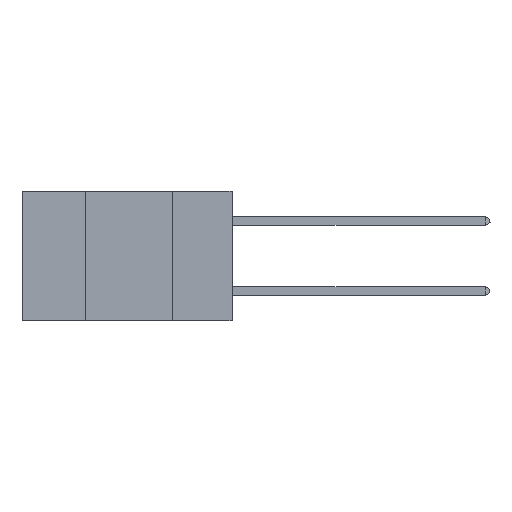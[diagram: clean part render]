
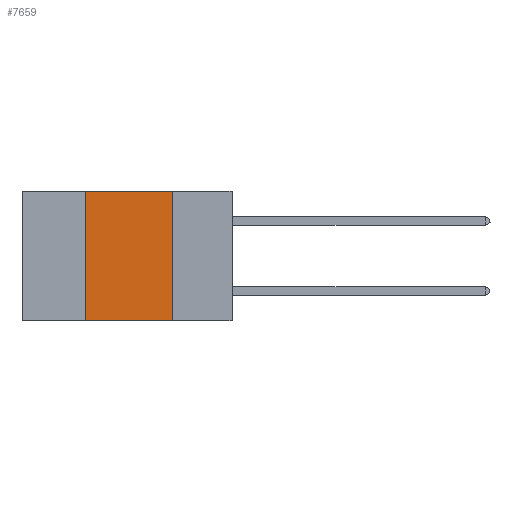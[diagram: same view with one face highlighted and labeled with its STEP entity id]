
A CAD part, left-side view. The second image highlights one B-rep face of the part: STEP entity #7659.
In plain terms, the highlighted planar face has unit normal (-1, 0, 0).
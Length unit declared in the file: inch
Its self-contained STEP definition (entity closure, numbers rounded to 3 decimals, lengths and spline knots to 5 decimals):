
#226 = DIRECTION ( 'NONE',  ( 0., 0., -1. ) ) ;
#374 = ORIENTED_EDGE ( 'NONE', *, *, #7671, .F. ) ;
#540 = VERTEX_POINT ( 'NONE', #12901 ) ;
#922 = EDGE_LOOP ( 'NONE', ( #374, #12411, #3783, #12778 ) ) ;
#1341 = LINE ( 'NONE', #3251, #9674 ) ;
#1402 = CARTESIAN_POINT ( 'NONE',  ( 0., 0.17, 0. ) ) ;
#3251 = CARTESIAN_POINT ( 'NONE',  ( 0., 0.42, 0. ) ) ;
#3254 = VECTOR ( 'NONE', #10732, 39.37008 ) ;
#3783 = ORIENTED_EDGE ( 'NONE', *, *, #9720, .F. ) ;
#4323 = DIRECTION ( 'NONE',  ( 0., 0., 1. ) ) ;
#4763 = DIRECTION ( 'NONE',  ( 1., 0., 0. ) ) ;
#4970 = VERTEX_POINT ( 'NONE', #5935 ) ;
#5128 = LINE ( 'NONE', #1402, #10412 ) ;
#5935 = CARTESIAN_POINT ( 'NONE',  ( 0., 0.17, 0. ) ) ;
#6244 = LINE ( 'NONE', #14028, #3254 ) ;
#6791 = CARTESIAN_POINT ( 'NONE',  ( 0., 0.6, 0. ) ) ;
#7073 = CARTESIAN_POINT ( 'NONE',  ( 0., 0.42, 0. ) ) ;
#7356 = CARTESIAN_POINT ( 'NONE',  ( 0., 0.42, -0.37 ) ) ;
#7659 = ADVANCED_FACE ( 'NONE', ( #13411 ), #11521, .F. ) ;
#7670 = VECTOR ( 'NONE', #11267, 39.37008 ) ;
#7671 = EDGE_CURVE ( 'NONE', #4970, #540, #5128, .T. ) ;
#7814 = VERTEX_POINT ( 'NONE', #7356 ) ;
#8778 = VERTEX_POINT ( 'NONE', #7073 ) ;
#9674 = VECTOR ( 'NONE', #4323, 39.37008 ) ;
#9720 = EDGE_CURVE ( 'NONE', #7814, #8778, #1341, .T. ) ;
#10387 = CARTESIAN_POINT ( 'NONE',  ( 0., 0.6, 0. ) ) ;
#10412 = VECTOR ( 'NONE', #226, 39.37008 ) ;
#10634 = LINE ( 'NONE', #6791, #7670 ) ;
#10732 = DIRECTION ( 'NONE',  ( 0., -1., 0. ) ) ;
#10953 = AXIS2_PLACEMENT_3D ( 'NONE', #10387, #4763, #12661 ) ;
#11267 = DIRECTION ( 'NONE',  ( 0., -1., 0. ) ) ;
#11521 = PLANE ( 'NONE',  #10953 ) ;
#12231 = EDGE_CURVE ( 'NONE', #7814, #540, #6244, .T. ) ;
#12411 = ORIENTED_EDGE ( 'NONE', *, *, #12581, .F. ) ;
#12581 = EDGE_CURVE ( 'NONE', #8778, #4970, #10634, .T. ) ;
#12661 = DIRECTION ( 'NONE',  ( 0., 0., -1. ) ) ;
#12778 = ORIENTED_EDGE ( 'NONE', *, *, #12231, .T. ) ;
#12901 = CARTESIAN_POINT ( 'NONE',  ( 0., 0.17, -0.37 ) ) ;
#13411 = FACE_OUTER_BOUND ( 'NONE', #922, .T. ) ;
#14028 = CARTESIAN_POINT ( 'NONE',  ( 0., 0.6, -0.37 ) ) ;
